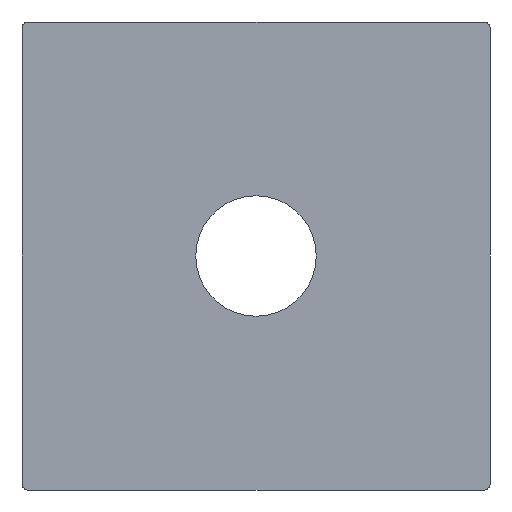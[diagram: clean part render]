
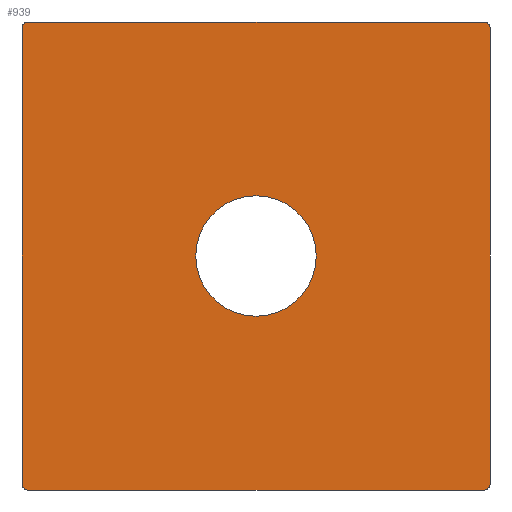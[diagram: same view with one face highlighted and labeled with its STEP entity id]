
A CAD part, front view. The second image highlights one B-rep face of the part: STEP entity #939.
In plain terms, the highlighted planar face has unit normal (0, -1, 0).
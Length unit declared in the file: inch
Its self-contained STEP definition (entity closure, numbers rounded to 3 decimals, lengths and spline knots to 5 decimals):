
#85=LINE('',#1467,#172);
#86=LINE('',#1469,#173);
#123=LINE('',#1681,#210);
#124=LINE('',#1683,#211);
#172=VECTOR('',#1184,0.3937);
#173=VECTOR('',#1187,0.3937);
#210=VECTOR('',#1310,0.3937);
#211=VECTOR('',#1313,0.3937);
#237=PLANE('',#1048);
#242=FACE_BOUND('',#359,.T.);
#298=FACE_OUTER_BOUND('',#358,.T.);
#358=EDGE_LOOP('',(#854,#855,#856,#857,#858,#859,#860,#861));
#359=EDGE_LOOP('',(#862));
#361=CIRCLE('',#962,0.2575);
#365=CIRCLE('',#979,0.025);
#369=CIRCLE('',#985,0.025);
#373=CIRCLE('',#991,0.025);
#377=CIRCLE('',#998,0.025);
#391=VERTEX_POINT('',#1320);
#417=VERTEX_POINT('',#1410);
#418=VERTEX_POINT('',#1411);
#422=VERTEX_POINT('',#1423);
#423=VERTEX_POINT('',#1424);
#427=VERTEX_POINT('',#1436);
#428=VERTEX_POINT('',#1437);
#432=VERTEX_POINT('',#1452);
#433=VERTEX_POINT('',#1453);
#471=EDGE_CURVE('',#391,#391,#361,.T.);
#508=EDGE_CURVE('',#417,#418,#365,.T.);
#514=EDGE_CURVE('',#422,#423,#369,.T.);
#520=EDGE_CURVE('',#427,#428,#373,.T.);
#528=EDGE_CURVE('',#432,#433,#377,.T.);
#537=EDGE_CURVE('',#417,#428,#85,.T.);
#538=EDGE_CURVE('',#427,#433,#86,.T.);
#599=EDGE_CURVE('',#422,#418,#123,.T.);
#600=EDGE_CURVE('',#432,#423,#124,.T.);
#854=ORIENTED_EDGE('',*,*,#508,.F.);
#855=ORIENTED_EDGE('',*,*,#537,.T.);
#856=ORIENTED_EDGE('',*,*,#520,.F.);
#857=ORIENTED_EDGE('',*,*,#538,.T.);
#858=ORIENTED_EDGE('',*,*,#528,.F.);
#859=ORIENTED_EDGE('',*,*,#600,.T.);
#860=ORIENTED_EDGE('',*,*,#514,.F.);
#861=ORIENTED_EDGE('',*,*,#599,.T.);
#862=ORIENTED_EDGE('',*,*,#471,.T.);
#939=ADVANCED_FACE('',(#298,#242),#237,.F.);
#962=AXIS2_PLACEMENT_3D('',#1321,#1055,#1056);
#979=AXIS2_PLACEMENT_3D('',#1412,#1120,#1121);
#985=AXIS2_PLACEMENT_3D('',#1425,#1134,#1135);
#991=AXIS2_PLACEMENT_3D('',#1438,#1148,#1149);
#998=AXIS2_PLACEMENT_3D('',#1454,#1166,#1167);
#1048=AXIS2_PLACEMENT_3D('',#1684,#1314,#1315);
#1055=DIRECTION('center_axis',(0.,1.,0.));
#1056=DIRECTION('ref_axis',(-1.,0.,0.));
#1120=DIRECTION('center_axis',(0.,1.,0.));
#1121=DIRECTION('ref_axis',(-0.707,0.,-0.707));
#1134=DIRECTION('center_axis',(0.,1.,0.));
#1135=DIRECTION('ref_axis',(-0.707,0.,0.707));
#1148=DIRECTION('center_axis',(0.,1.,0.));
#1149=DIRECTION('ref_axis',(0.707,0.,-0.707));
#1166=DIRECTION('center_axis',(0.,1.,0.));
#1167=DIRECTION('ref_axis',(0.707,0.,0.707));
#1184=DIRECTION('',(1.,0.,0.));
#1187=DIRECTION('',(0.,0.,1.));
#1310=DIRECTION('',(0.,0.,-1.));
#1313=DIRECTION('',(-1.,0.,0.));
#1314=DIRECTION('center_axis',(0.,1.,0.));
#1315=DIRECTION('ref_axis',(0.,0.,1.));
#1320=CARTESIAN_POINT('',(-0.7425,0.,-1.));
#1321=CARTESIAN_POINT('Origin',(-1.,0.,-1.));
#1410=CARTESIAN_POINT('',(-1.975,0.,-2.));
#1411=CARTESIAN_POINT('',(-2.,0.,-1.975));
#1412=CARTESIAN_POINT('Origin',(-1.975,0.,-1.975));
#1423=CARTESIAN_POINT('',(-2.,0.,-0.025));
#1424=CARTESIAN_POINT('',(-1.975,0.,0.));
#1425=CARTESIAN_POINT('Origin',(-1.975,0.,-0.025));
#1436=CARTESIAN_POINT('',(0.,0.,-1.975));
#1437=CARTESIAN_POINT('',(-0.025,0.,-2.));
#1438=CARTESIAN_POINT('Origin',(-0.025,0.,-1.975));
#1452=CARTESIAN_POINT('',(-0.025,0.,0.));
#1453=CARTESIAN_POINT('',(0.,0.,-0.025));
#1454=CARTESIAN_POINT('Origin',(-0.025,0.,-0.025));
#1467=CARTESIAN_POINT('',(-2.,0.,-2.));
#1469=CARTESIAN_POINT('',(0.,0.,-2.));
#1681=CARTESIAN_POINT('',(-2.,0.,0.));
#1683=CARTESIAN_POINT('',(0.,0.,0.));
#1684=CARTESIAN_POINT('Origin',(-1.,0.,-1.));
